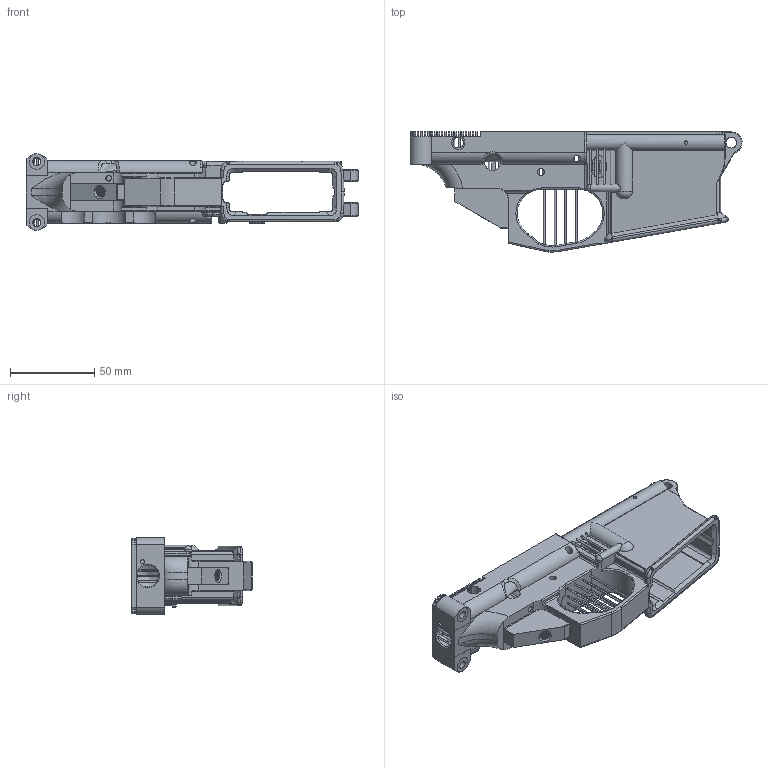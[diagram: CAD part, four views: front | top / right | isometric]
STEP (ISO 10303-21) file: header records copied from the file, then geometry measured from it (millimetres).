
FILE_DESCRIPTION(/* description */ ('Alibre Inc.'),/* implementation_level */ '2;1');
FILE_NAME(/* name */ 'export0',/* time_stamp */ '2015-10-03T20:30:27-07:00',/* author */ (''),/* organization */ (''),/* preprocessor_version */ 'ST-DEVELOPER v14',/* originating_system */ 'Alibre',/* authorisation */ '');
FILE_SCHEMA (('AUTOMOTIVE_DESIGN'));
Length unit declared in the file: inch
Bounding box: 196.91 x 71.26 x 45.46 mm (x, y, z)
Volume: 123236.9 mm3; surface area: 73476.2 mm2
Topology: 76 solids, 123 shells, 1850 faces, 4718 edges, 3130 vertices
Faces by surface type: plane 781, cylinder 733, bspline 187, cone 96, torus 47, sphere 6
Full cylindrical faces by diameter (mm): 0.051 x149, 1.067 x161, 1.981 x1, 2.362 x2, 2.388 x1, 2.464 x1, 3.175 x1, 3.937 x4, 3.969 x5, 4.056 x32, 4.826 x30, 5.182 x1, 6.375 x4, 6.477 x1, 7.938 x1, 9.169 x2, 9.525 x3, 12.7 x1
Entity records: 80291 total; most frequent: CARTESIAN_POINT 42545, ORIENTED_EDGE 8206, DIRECTION 5695, EDGE_CURVE 4103, VERTEX_POINT 3000, FACE_BOUND 2687, EDGE_LOOP 2684, AXIS2_PLACEMENT_3D 2402
